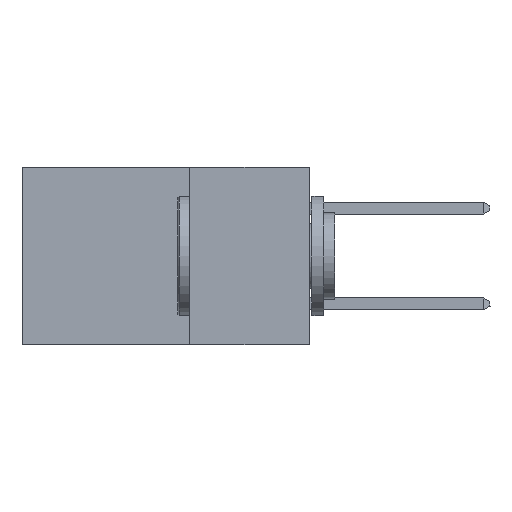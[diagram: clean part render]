
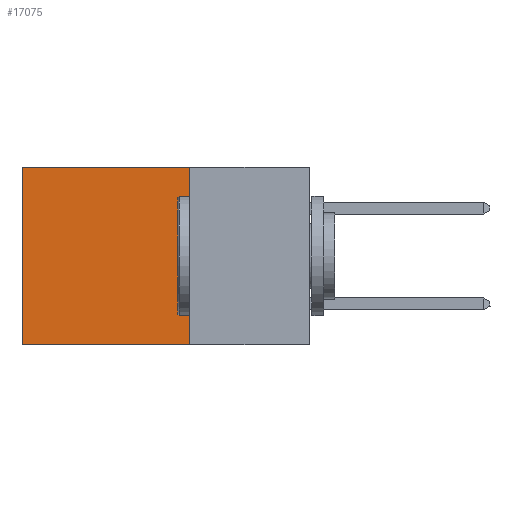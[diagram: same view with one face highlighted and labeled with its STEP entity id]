
A CAD part, left-side view. The second image highlights one B-rep face of the part: STEP entity #17075.
In plain terms, the highlighted planar face has unit normal (-1, 0, 0).
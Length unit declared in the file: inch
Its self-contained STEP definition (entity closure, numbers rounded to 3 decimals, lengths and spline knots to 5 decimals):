
#214 = CARTESIAN_POINT ( 'NONE',  ( 0.2875, 0.25, 0. ) ) ;
#432 = ORIENTED_EDGE ( 'NONE', *, *, #17969, .F. ) ;
#650 = VERTEX_POINT ( 'NONE', #8273 ) ;
#765 = CARTESIAN_POINT ( 'NONE',  ( 0.2875, 0.25, -0.37 ) ) ;
#994 = VERTEX_POINT ( 'NONE', #214 ) ;
#1206 = CARTESIAN_POINT ( 'NONE',  ( 0.2875, 0.25, 0. ) ) ;
#1775 = EDGE_CURVE ( 'NONE', #994, #650, #14266, .T. ) ;
#1914 = ORIENTED_EDGE ( 'NONE', *, *, #12403, .T. ) ;
#4324 = FACE_OUTER_BOUND ( 'NONE', #17500, .T. ) ;
#4432 = DIRECTION ( 'NONE',  ( 0., 0., -1. ) ) ;
#5036 = VECTOR ( 'NONE', #6043, 39.37008 ) ;
#5585 = DIRECTION ( 'NONE',  ( 0., 0., -1. ) ) ;
#6028 = VECTOR ( 'NONE', #5585, 39.37008 ) ;
#6043 = DIRECTION ( 'NONE',  ( 0., 0., -1. ) ) ;
#7487 = CARTESIAN_POINT ( 'NONE',  ( 0.2875, 0.25, 0. ) ) ;
#7678 = DIRECTION ( 'NONE',  ( 0., 1., 0. ) ) ;
#7689 = EDGE_CURVE ( 'NONE', #8586, #16117, #17898, .T. ) ;
#8273 = CARTESIAN_POINT ( 'NONE',  ( 0.2875, 0.6, 0. ) ) ;
#8389 = CARTESIAN_POINT ( 'NONE',  ( 0.2875, 0.6, -0.37 ) ) ;
#8586 = VERTEX_POINT ( 'NONE', #765 ) ;
#8782 = DIRECTION ( 'NONE',  ( 0., 1., 0. ) ) ;
#10895 = CARTESIAN_POINT ( 'NONE',  ( 0.2875, 0.25, 0. ) ) ;
#12403 = EDGE_CURVE ( 'NONE', #650, #16117, #13997, .T. ) ;
#13958 = DIRECTION ( 'NONE',  ( 1., 0., 0. ) ) ;
#13981 = LINE ( 'NONE', #10895, #5036 ) ;
#13997 = LINE ( 'NONE', #19776, #6028 ) ;
#14266 = LINE ( 'NONE', #7487, #17992 ) ;
#14548 = AXIS2_PLACEMENT_3D ( 'NONE', #1206, #13958, #4432 ) ;
#14940 = VECTOR ( 'NONE', #7678, 39.37008 ) ;
#15593 = CARTESIAN_POINT ( 'NONE',  ( 0.2875, 0.25, -0.37 ) ) ;
#16011 = ORIENTED_EDGE ( 'NONE', *, *, #1775, .T. ) ;
#16117 = VERTEX_POINT ( 'NONE', #8389 ) ;
#17075 = ADVANCED_FACE ( 'NONE', ( #4324 ), #20083, .F. ) ;
#17500 = EDGE_LOOP ( 'NONE', ( #1914, #18391, #432, #16011 ) ) ;
#17898 = LINE ( 'NONE', #15593, #14940 ) ;
#17969 = EDGE_CURVE ( 'NONE', #994, #8586, #13981, .T. ) ;
#17992 = VECTOR ( 'NONE', #8782, 39.37008 ) ;
#18391 = ORIENTED_EDGE ( 'NONE', *, *, #7689, .F. ) ;
#19776 = CARTESIAN_POINT ( 'NONE',  ( 0.2875, 0.6, 0. ) ) ;
#20083 = PLANE ( 'NONE',  #14548 ) ;
